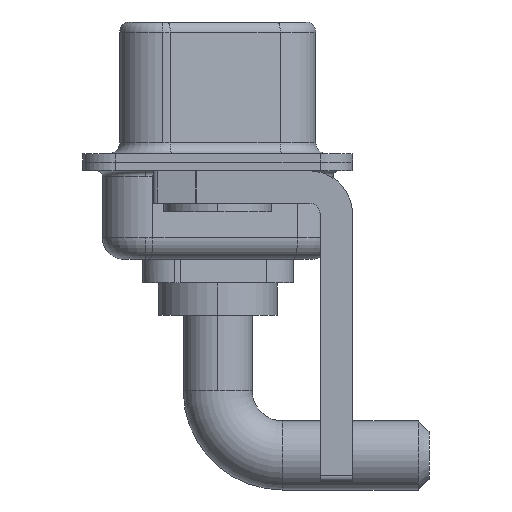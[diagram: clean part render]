
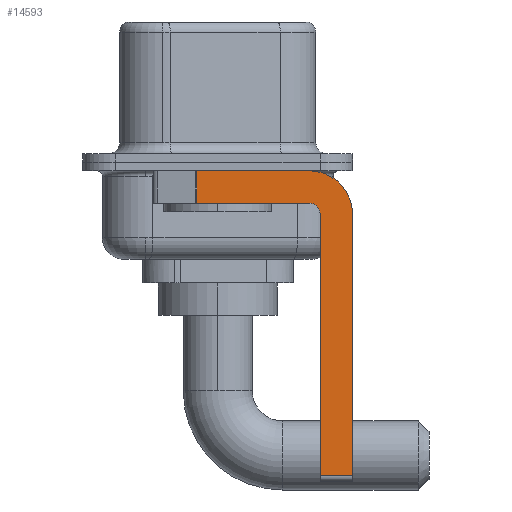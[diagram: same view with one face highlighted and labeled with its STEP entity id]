
A CAD part, left-side view. The second image highlights one B-rep face of the part: STEP entity #14593.
In plain terms, the highlighted planar face has unit normal (-1, 0, 0).
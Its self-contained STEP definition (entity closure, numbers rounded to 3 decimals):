
#276 = VECTOR ( 'NONE', #2290, 1000. ) ;
#419 = ORIENTED_EDGE ( 'NONE', *, *, #2591, .F. ) ;
#619 = DIRECTION ( 'NONE',  ( 0., 0., -1. ) ) ;
#647 = CARTESIAN_POINT ( 'NONE',  ( -2.9, -4.25, -0.4 ) ) ;
#842 = CARTESIAN_POINT ( 'NONE',  ( -2.9, 0.978, -1.9 ) ) ;
#1019 = VERTEX_POINT ( 'NONE', #7085 ) ;
#1631 = EDGE_CURVE ( 'NONE', #13602, #11655, #14675, .T. ) ;
#1737 = VECTOR ( 'NONE', #3955, 1000. ) ;
#1830 = ORIENTED_EDGE ( 'NONE', *, *, #7637, .F. ) ;
#2062 = DIRECTION ( 'NONE',  ( 0., -1., 0. ) ) ;
#2290 = DIRECTION ( 'NONE',  ( 0., 0., -1. ) ) ;
#2332 = VERTEX_POINT ( 'NONE', #11248 ) ;
#2390 = VECTOR ( 'NONE', #2062, 1000. ) ;
#2591 = EDGE_CURVE ( 'NONE', #11655, #1019, #6170, .T. ) ;
#2624 = CARTESIAN_POINT ( 'NONE',  ( -2.9, -6.25, -2.4 ) ) ;
#2917 = CARTESIAN_POINT ( 'NONE',  ( -2.9, -6.25, -14.55 ) ) ;
#3563 = AXIS2_PLACEMENT_3D ( 'NONE', #14821, #9130, #13993 ) ;
#3736 = DIRECTION ( 'NONE',  ( 0., 0., 1. ) ) ;
#3835 = LINE ( 'NONE', #8508, #7716 ) ;
#3955 = DIRECTION ( 'NONE',  ( 0., 1., 0. ) ) ;
#4096 = CARTESIAN_POINT ( 'NONE',  ( -2.9, -4.25, -1.9 ) ) ;
#4400 = VERTEX_POINT ( 'NONE', #9694 ) ;
#4762 = EDGE_CURVE ( 'NONE', #2332, #14204, #7281, .T. ) ;
#4883 = DIRECTION ( 'NONE',  ( 1., 0., 0. ) ) ;
#5942 = LINE ( 'NONE', #9635, #12472 ) ;
#6091 = CARTESIAN_POINT ( 'NONE',  ( -2.9, -4.75, -2.4 ) ) ;
#6111 = EDGE_CURVE ( 'NONE', #11922, #7092, #12589, .T. ) ;
#6170 = LINE ( 'NONE', #4096, #1737 ) ;
#6726 = LINE ( 'NONE', #842, #276 ) ;
#7085 = CARTESIAN_POINT ( 'NONE',  ( -2.9, 0.978, -1.9 ) ) ;
#7092 = VERTEX_POINT ( 'NONE', #647 ) ;
#7258 = FACE_OUTER_BOUND ( 'NONE', #14236, .T. ) ;
#7281 = LINE ( 'NONE', #2624, #14338 ) ;
#7637 = EDGE_CURVE ( 'NONE', #7092, #2332, #8211, .T. ) ;
#7716 = VECTOR ( 'NONE', #9590, 1000. ) ;
#8098 = ORIENTED_EDGE ( 'NONE', *, *, #4762, .F. ) ;
#8211 = CIRCLE ( 'NONE', #3563, 2. ) ;
#8263 = CARTESIAN_POINT ( 'NONE',  ( -2.9, -4.25, -2.4 ) ) ;
#8418 = PLANE ( 'NONE',  #10842 ) ;
#8508 = CARTESIAN_POINT ( 'NONE',  ( -2.9, -4.25, -14.55 ) ) ;
#9130 = DIRECTION ( 'NONE',  ( 1., 0., 0. ) ) ;
#9347 = ORIENTED_EDGE ( 'NONE', *, *, #9428, .T. ) ;
#9428 = EDGE_CURVE ( 'NONE', #4400, #14204, #3835, .T. ) ;
#9552 = CARTESIAN_POINT ( 'NONE',  ( -2.9, -4.25, -1.9 ) ) ;
#9590 = DIRECTION ( 'NONE',  ( 0., -1., 0. ) ) ;
#9635 = CARTESIAN_POINT ( 'NONE',  ( -2.9, -4.75, -14.8 ) ) ;
#9694 = CARTESIAN_POINT ( 'NONE',  ( -2.9, -4.75, -14.55 ) ) ;
#9898 = CARTESIAN_POINT ( 'NONE',  ( -2.9, -4.25, -2.4 ) ) ;
#10119 = CARTESIAN_POINT ( 'NONE',  ( -2.9, 3., -0.4 ) ) ;
#10125 = DIRECTION ( 'NONE',  ( -1., 0., 0. ) ) ;
#10343 = ORIENTED_EDGE ( 'NONE', *, *, #6111, .F. ) ;
#10783 = AXIS2_PLACEMENT_3D ( 'NONE', #9898, #10125, #14805 ) ;
#10842 = AXIS2_PLACEMENT_3D ( 'NONE', #8263, #4883, #11976 ) ;
#11124 = ORIENTED_EDGE ( 'NONE', *, *, #14440, .T. ) ;
#11248 = CARTESIAN_POINT ( 'NONE',  ( -2.9, -6.25, -2.4 ) ) ;
#11430 = ORIENTED_EDGE ( 'NONE', *, *, #1631, .F. ) ;
#11655 = VERTEX_POINT ( 'NONE', #9552 ) ;
#11669 = EDGE_CURVE ( 'NONE', #4400, #13602, #5942, .T. ) ;
#11921 = ORIENTED_EDGE ( 'NONE', *, *, #11669, .F. ) ;
#11922 = VERTEX_POINT ( 'NONE', #12559 ) ;
#11976 = DIRECTION ( 'NONE',  ( 0., 0., -1. ) ) ;
#12472 = VECTOR ( 'NONE', #3736, 1000. ) ;
#12559 = CARTESIAN_POINT ( 'NONE',  ( -2.9, 0.978, -0.4 ) ) ;
#12589 = LINE ( 'NONE', #10119, #2390 ) ;
#13602 = VERTEX_POINT ( 'NONE', #6091 ) ;
#13993 = DIRECTION ( 'NONE',  ( 0., 0., -1. ) ) ;
#14204 = VERTEX_POINT ( 'NONE', #2917 ) ;
#14236 = EDGE_LOOP ( 'NONE', ( #10343, #11124, #419, #11430, #11921, #9347, #8098, #1830 ) ) ;
#14338 = VECTOR ( 'NONE', #619, 1000. ) ;
#14440 = EDGE_CURVE ( 'NONE', #11922, #1019, #6726, .T. ) ;
#14593 = ADVANCED_FACE ( 'NONE', ( #7258 ), #8418, .F. ) ;
#14675 = CIRCLE ( 'NONE', #10783, 0.5 ) ;
#14805 = DIRECTION ( 'NONE',  ( 0., 0., 1. ) ) ;
#14821 = CARTESIAN_POINT ( 'NONE',  ( -2.9, -4.25, -2.4 ) ) ;
